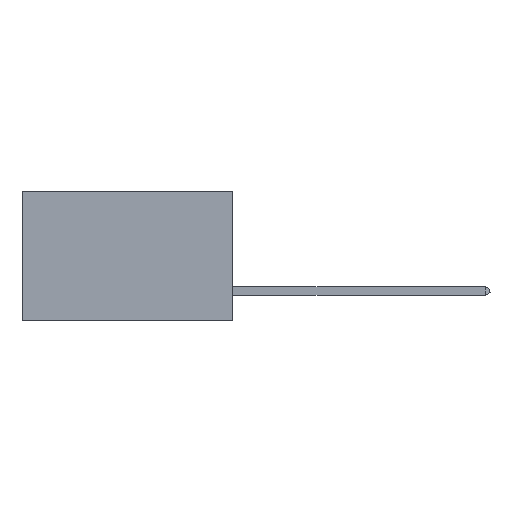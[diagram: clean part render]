
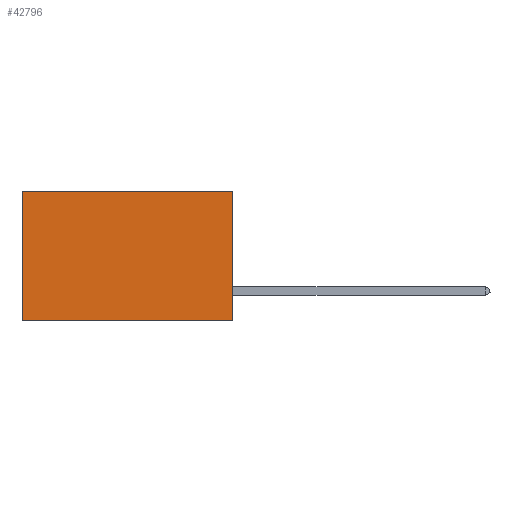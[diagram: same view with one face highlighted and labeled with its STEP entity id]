
A CAD part, left-side view. The second image highlights one B-rep face of the part: STEP entity #42796.
In plain terms, the highlighted planar face has unit normal (-1, 0, 0).
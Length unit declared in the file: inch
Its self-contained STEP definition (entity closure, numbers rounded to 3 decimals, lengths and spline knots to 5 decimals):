
#256 = VERTEX_POINT ( 'NONE', #12845 ) ;
#339 = DIRECTION ( 'NONE',  ( 0., 1., 0. ) ) ;
#1056 = CARTESIAN_POINT ( 'NONE',  ( 0.2875, 0., 0. ) ) ;
#4134 = EDGE_CURVE ( 'NONE', #34419, #256, #22191, .T. ) ;
#4658 = CARTESIAN_POINT ( 'NONE',  ( 0.2875, 0., -0.37 ) ) ;
#8460 = LINE ( 'NONE', #22222, #43394 ) ;
#8867 = DIRECTION ( 'NONE',  ( 0., 1., 0. ) ) ;
#9132 = VERTEX_POINT ( 'NONE', #4658 ) ;
#10925 = ORIENTED_EDGE ( 'NONE', *, *, #23004, .T. ) ;
#12845 = CARTESIAN_POINT ( 'NONE',  ( 0.2875, 0.6, 0. ) ) ;
#13246 = VECTOR ( 'NONE', #339, 39.37008 ) ;
#14744 = PLANE ( 'NONE',  #40800 ) ;
#15059 = ORIENTED_EDGE ( 'NONE', *, *, #32051, .F. ) ;
#18878 = ORIENTED_EDGE ( 'NONE', *, *, #39969, .F. ) ;
#19146 = CARTESIAN_POINT ( 'NONE',  ( 0.2875, 0., 0. ) ) ;
#19368 = CARTESIAN_POINT ( 'NONE',  ( 0.2875, 0., -0.37 ) ) ;
#22191 = LINE ( 'NONE', #34177, #13246 ) ;
#22222 = CARTESIAN_POINT ( 'NONE',  ( 0.2875, 0.6, 0. ) ) ;
#22400 = VERTEX_POINT ( 'NONE', #25278 ) ;
#23004 = EDGE_CURVE ( 'NONE', #256, #22400, #8460, .T. ) ;
#23365 = VECTOR ( 'NONE', #42132, 39.37008 ) ;
#23403 = EDGE_LOOP ( 'NONE', ( #10925, #18878, #15059, #25656 ) ) ;
#25278 = CARTESIAN_POINT ( 'NONE',  ( 0.2875, 0.6, -0.37 ) ) ;
#25656 = ORIENTED_EDGE ( 'NONE', *, *, #4134, .T. ) ;
#25771 = DIRECTION ( 'NONE',  ( 0., 0., -1. ) ) ;
#27823 = DIRECTION ( 'NONE',  ( 1., 0., 0. ) ) ;
#30945 = LINE ( 'NONE', #19368, #42109 ) ;
#31276 = DIRECTION ( 'NONE',  ( 0., 0., -1. ) ) ;
#31912 = CARTESIAN_POINT ( 'NONE',  ( 0.2875, 0., 0. ) ) ;
#32051 = EDGE_CURVE ( 'NONE', #34419, #9132, #40806, .T. ) ;
#34177 = CARTESIAN_POINT ( 'NONE',  ( 0.2875, 0., 0. ) ) ;
#34419 = VERTEX_POINT ( 'NONE', #19146 ) ;
#34436 = FACE_OUTER_BOUND ( 'NONE', #23403, .T. ) ;
#39969 = EDGE_CURVE ( 'NONE', #9132, #22400, #30945, .T. ) ;
#40800 = AXIS2_PLACEMENT_3D ( 'NONE', #31912, #27823, #31276 ) ;
#40806 = LINE ( 'NONE', #1056, #23365 ) ;
#42109 = VECTOR ( 'NONE', #8867, 39.37008 ) ;
#42132 = DIRECTION ( 'NONE',  ( 0., 0., -1. ) ) ;
#42796 = ADVANCED_FACE ( 'NONE', ( #34436 ), #14744, .F. ) ;
#43394 = VECTOR ( 'NONE', #25771, 39.37008 ) ;
